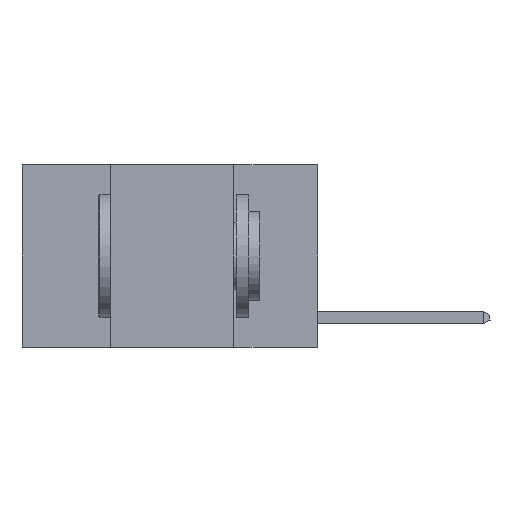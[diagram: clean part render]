
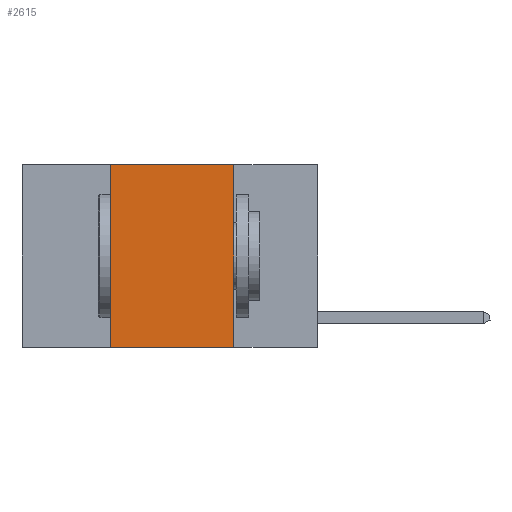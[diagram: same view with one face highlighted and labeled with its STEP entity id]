
A CAD part, left-side view. The second image highlights one B-rep face of the part: STEP entity #2615.
In plain terms, the highlighted planar face has unit normal (-1, 0, 0).
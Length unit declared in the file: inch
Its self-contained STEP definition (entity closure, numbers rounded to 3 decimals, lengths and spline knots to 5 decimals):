
#1668 = CARTESIAN_POINT ( 'NONE',  ( 0., 0.6, -0.37 ) ) ;
#1767 = EDGE_LOOP ( 'NONE', ( #18531, #22144, #8965, #17960 ) ) ;
#2349 = CARTESIAN_POINT ( 'NONE',  ( 0., 0.42, -0.37 ) ) ;
#2360 = DIRECTION ( 'NONE',  ( 1., 0., 0. ) ) ;
#2509 = LINE ( 'NONE', #9293, #7987 ) ;
#2615 = ADVANCED_FACE ( 'NONE', ( #12934 ), #14833, .F. ) ;
#2827 = EDGE_CURVE ( 'NONE', #25979, #12587, #2509, .T. ) ;
#7927 = AXIS2_PLACEMENT_3D ( 'NONE', #12717, #2360, #16904 ) ;
#7987 = VECTOR ( 'NONE', #11417, 39.37008 ) ;
#8965 = ORIENTED_EDGE ( 'NONE', *, *, #13468, .F. ) ;
#8993 = CARTESIAN_POINT ( 'NONE',  ( 0., 0.17, 0. ) ) ;
#9170 = CARTESIAN_POINT ( 'NONE',  ( 0., 0.42, 0. ) ) ;
#9293 = CARTESIAN_POINT ( 'NONE',  ( 0., 0.6, 0. ) ) ;
#10510 = CARTESIAN_POINT ( 'NONE',  ( 0., 0.42, 0. ) ) ;
#10945 = VERTEX_POINT ( 'NONE', #2349 ) ;
#11129 = DIRECTION ( 'NONE',  ( 0., 0., -1. ) ) ;
#11417 = DIRECTION ( 'NONE',  ( 0., -1., 0. ) ) ;
#11813 = CARTESIAN_POINT ( 'NONE',  ( 0., 0.17, 0. ) ) ;
#11942 = EDGE_CURVE ( 'NONE', #10945, #13535, #23416, .T. ) ;
#12587 = VERTEX_POINT ( 'NONE', #11813 ) ;
#12717 = CARTESIAN_POINT ( 'NONE',  ( 0., 0.6, 0. ) ) ;
#12854 = CARTESIAN_POINT ( 'NONE',  ( 0., 0.17, -0.37 ) ) ;
#12934 = FACE_OUTER_BOUND ( 'NONE', #1767, .T. ) ;
#13468 = EDGE_CURVE ( 'NONE', #10945, #25979, #13943, .T. ) ;
#13535 = VERTEX_POINT ( 'NONE', #12854 ) ;
#13943 = LINE ( 'NONE', #10510, #21393 ) ;
#14833 = PLANE ( 'NONE',  #7927 ) ;
#15029 = VECTOR ( 'NONE', #16208, 39.37008 ) ;
#16128 = VECTOR ( 'NONE', #11129, 39.37008 ) ;
#16208 = DIRECTION ( 'NONE',  ( 0., -1., 0. ) ) ;
#16904 = DIRECTION ( 'NONE',  ( 0., 0., -1. ) ) ;
#17960 = ORIENTED_EDGE ( 'NONE', *, *, #11942, .T. ) ;
#18531 = ORIENTED_EDGE ( 'NONE', *, *, #20231, .F. ) ;
#20231 = EDGE_CURVE ( 'NONE', #12587, #13535, #21633, .T. ) ;
#21393 = VECTOR ( 'NONE', #22937, 39.37008 ) ;
#21633 = LINE ( 'NONE', #8993, #16128 ) ;
#22144 = ORIENTED_EDGE ( 'NONE', *, *, #2827, .F. ) ;
#22937 = DIRECTION ( 'NONE',  ( 0., 0., 1. ) ) ;
#23416 = LINE ( 'NONE', #1668, #15029 ) ;
#25979 = VERTEX_POINT ( 'NONE', #9170 ) ;
